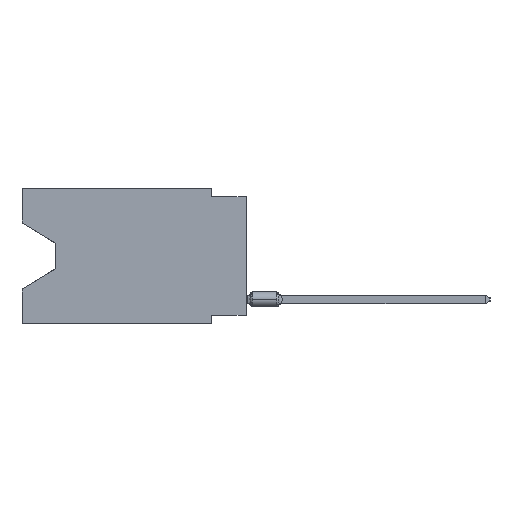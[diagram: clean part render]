
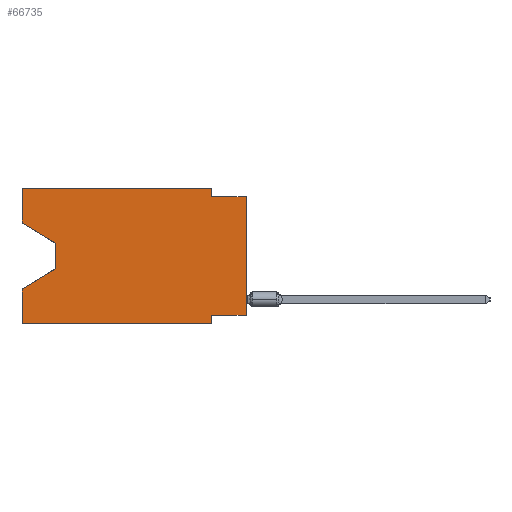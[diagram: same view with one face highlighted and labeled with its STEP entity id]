
A CAD part, left-side view. The second image highlights one B-rep face of the part: STEP entity #66735.
In plain terms, the highlighted planar face has unit normal (-1, 0, 0).
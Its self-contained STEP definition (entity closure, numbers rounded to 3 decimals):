
#975 = CARTESIAN_POINT ( 'NONE',  ( 0., 16.383, -9.906 ) ) ;
#2247 = VERTEX_POINT ( 'NONE', #31099 ) ;
#2841 = ORIENTED_EDGE ( 'NONE', *, *, #19397, .F. ) ;
#3547 = VECTOR ( 'NONE', #15946, 1000. ) ;
#5544 = VERTEX_POINT ( 'NONE', #37851 ) ;
#6447 = CARTESIAN_POINT ( 'NONE',  ( 0., 16.383, 0. ) ) ;
#9042 = LINE ( 'NONE', #21674, #3547 ) ;
#9742 = EDGE_CURVE ( 'NONE', #5544, #59320, #74086, .T. ) ;
#12204 = FACE_OUTER_BOUND ( 'NONE', #25759, .T. ) ;
#13339 = ORIENTED_EDGE ( 'NONE', *, *, #69992, .F. ) ;
#13343 = CARTESIAN_POINT ( 'NONE',  ( 0., 2.54, 0. ) ) ;
#15040 = DIRECTION ( 'NONE',  ( 0., 0., 1. ) ) ;
#15249 = CARTESIAN_POINT ( 'NONE',  ( 0., 16.383, -2.546 ) ) ;
#15946 = DIRECTION ( 'NONE',  ( 0., -1., 0. ) ) ;
#18951 = EDGE_CURVE ( 'NONE', #69883, #52022, #30192, .T. ) ;
#19292 = CARTESIAN_POINT ( 'NONE',  ( 0., 16.383, -2.546 ) ) ;
#19304 = VECTOR ( 'NONE', #20701, 1000. ) ;
#19397 = EDGE_CURVE ( 'NONE', #34182, #2247, #49482, .T. ) ;
#19448 = CARTESIAN_POINT ( 'NONE',  ( 0., 0., 0. ) ) ;
#20510 = CARTESIAN_POINT ( 'NONE',  ( 0., 16.383, 0. ) ) ;
#20682 = VECTOR ( 'NONE', #36139, 1000. ) ;
#20701 = DIRECTION ( 'NONE',  ( 0., 0.855, -0.519 ) ) ;
#21674 = CARTESIAN_POINT ( 'NONE',  ( 0., 16.383, 0. ) ) ;
#22141 = VECTOR ( 'NONE', #64685, 1000. ) ;
#22697 = ORIENTED_EDGE ( 'NONE', *, *, #55579, .F. ) ;
#23872 = VECTOR ( 'NONE', #60016, 1000. ) ;
#23886 = CARTESIAN_POINT ( 'NONE',  ( 0., 2.54, -9.906 ) ) ;
#24367 = DIRECTION ( 'NONE',  ( 0., -1., 0. ) ) ;
#25759 = EDGE_LOOP ( 'NONE', ( #30781, #75148, #58285, #2841, #42229, #50373, #13339, #27452, #71503, #27538, #65998, #22697 ) ) ;
#25778 = CARTESIAN_POINT ( 'NONE',  ( 0., 16.383, 0. ) ) ;
#26527 = DIRECTION ( 'NONE',  ( 0., 0., 1. ) ) ;
#27452 = ORIENTED_EDGE ( 'NONE', *, *, #18951, .T. ) ;
#27538 = ORIENTED_EDGE ( 'NONE', *, *, #59784, .F. ) ;
#27880 = CARTESIAN_POINT ( 'NONE',  ( 0., 0., -9.271 ) ) ;
#27900 = EDGE_CURVE ( 'NONE', #73629, #42611, #9042, .T. ) ;
#29206 = VECTOR ( 'NONE', #29652, 1000. ) ;
#29652 = DIRECTION ( 'NONE',  ( 0., -0.855, -0.519 ) ) ;
#29824 = DIRECTION ( 'NONE',  ( 1., 0., 0. ) ) ;
#29923 = CARTESIAN_POINT ( 'NONE',  ( 0., 0., -0.635 ) ) ;
#30035 = LINE ( 'NONE', #19292, #29206 ) ;
#30192 = LINE ( 'NONE', #19448, #43479 ) ;
#30781 = ORIENTED_EDGE ( 'NONE', *, *, #48621, .T. ) ;
#31099 = CARTESIAN_POINT ( 'NONE',  ( 0., 16.383, -7.36 ) ) ;
#31426 = CARTESIAN_POINT ( 'NONE',  ( 0., 13.97, -5.893 ) ) ;
#32023 = CARTESIAN_POINT ( 'NONE',  ( 0., 2.54, 0. ) ) ;
#34182 = VERTEX_POINT ( 'NONE', #67827 ) ;
#34357 = CARTESIAN_POINT ( 'NONE',  ( 0., 2.54, -9.906 ) ) ;
#35885 = DIRECTION ( 'NONE',  ( 0., 1., 0. ) ) ;
#36139 = DIRECTION ( 'NONE',  ( 0., 0., -1. ) ) ;
#37851 = CARTESIAN_POINT ( 'NONE',  ( 0., 13.97, -4.013 ) ) ;
#38012 = EDGE_CURVE ( 'NONE', #70819, #52022, #75095, .T. ) ;
#38298 = LINE ( 'NONE', #31426, #19304 ) ;
#39870 = VECTOR ( 'NONE', #15040, 1000. ) ;
#41022 = CARTESIAN_POINT ( 'NONE',  ( 0., 2.54, -9.271 ) ) ;
#41683 = DIRECTION ( 'NONE',  ( 0., 0., -1. ) ) ;
#41801 = EDGE_CURVE ( 'NONE', #34182, #57193, #59590, .T. ) ;
#42010 = CARTESIAN_POINT ( 'NONE',  ( 0., 0., -9.271 ) ) ;
#42229 = ORIENTED_EDGE ( 'NONE', *, *, #41801, .T. ) ;
#42611 = VERTEX_POINT ( 'NONE', #13343 ) ;
#43479 = VECTOR ( 'NONE', #48913, 1000. ) ;
#46321 = CARTESIAN_POINT ( 'NONE',  ( 0., 13.97, -5.893 ) ) ;
#46770 = VECTOR ( 'NONE', #24367, 1000. ) ;
#48500 = LINE ( 'NONE', #42010, #48800 ) ;
#48554 = EDGE_CURVE ( 'NONE', #68034, #57193, #65264, .T. ) ;
#48621 = EDGE_CURVE ( 'NONE', #73162, #5544, #30035, .T. ) ;
#48725 = CARTESIAN_POINT ( 'NONE',  ( 0., 16.383, 0. ) ) ;
#48800 = VECTOR ( 'NONE', #35885, 1000. ) ;
#48913 = DIRECTION ( 'NONE',  ( 0., 0., 1. ) ) ;
#49482 = LINE ( 'NONE', #48725, #39870 ) ;
#50373 = ORIENTED_EDGE ( 'NONE', *, *, #48554, .F. ) ;
#51043 = CARTESIAN_POINT ( 'NONE',  ( 0., 13.97, -4.013 ) ) ;
#52022 = VERTEX_POINT ( 'NONE', #29923 ) ;
#55008 = LINE ( 'NONE', #32023, #23872 ) ;
#55579 = EDGE_CURVE ( 'NONE', #73162, #73629, #60625, .T. ) ;
#57193 = VERTEX_POINT ( 'NONE', #34357 ) ;
#58285 = ORIENTED_EDGE ( 'NONE', *, *, #68229, .T. ) ;
#58918 = PLANE ( 'NONE',  #68091 ) ;
#59320 = VERTEX_POINT ( 'NONE', #46321 ) ;
#59590 = LINE ( 'NONE', #975, #46770 ) ;
#59784 = EDGE_CURVE ( 'NONE', #42611, #70819, #55008, .T. ) ;
#60016 = DIRECTION ( 'NONE',  ( 0., 0., -1. ) ) ;
#60625 = LINE ( 'NONE', #25778, #70172 ) ;
#63559 = CARTESIAN_POINT ( 'NONE',  ( 0., 0., -0.635 ) ) ;
#64685 = DIRECTION ( 'NONE',  ( 0., -1., 0. ) ) ;
#65194 = CARTESIAN_POINT ( 'NONE',  ( 0., 2.54, -0.635 ) ) ;
#65264 = LINE ( 'NONE', #23886, #20682 ) ;
#65998 = ORIENTED_EDGE ( 'NONE', *, *, #27900, .F. ) ;
#66735 = ADVANCED_FACE ( 'NONE', ( #12204 ), #58918, .F. ) ;
#67827 = CARTESIAN_POINT ( 'NONE',  ( 0., 16.383, -9.906 ) ) ;
#68034 = VERTEX_POINT ( 'NONE', #41022 ) ;
#68091 = AXIS2_PLACEMENT_3D ( 'NONE', #6447, #29824, #41683 ) ;
#68229 = EDGE_CURVE ( 'NONE', #59320, #2247, #38298, .T. ) ;
#68329 = VECTOR ( 'NONE', #74470, 1000. ) ;
#69883 = VERTEX_POINT ( 'NONE', #27880 ) ;
#69992 = EDGE_CURVE ( 'NONE', #69883, #68034, #48500, .T. ) ;
#70172 = VECTOR ( 'NONE', #26527, 1000. ) ;
#70819 = VERTEX_POINT ( 'NONE', #65194 ) ;
#71503 = ORIENTED_EDGE ( 'NONE', *, *, #38012, .F. ) ;
#73162 = VERTEX_POINT ( 'NONE', #15249 ) ;
#73629 = VERTEX_POINT ( 'NONE', #20510 ) ;
#74086 = LINE ( 'NONE', #51043, #68329 ) ;
#74470 = DIRECTION ( 'NONE',  ( 0., 0., -1. ) ) ;
#75095 = LINE ( 'NONE', #63559, #22141 ) ;
#75148 = ORIENTED_EDGE ( 'NONE', *, *, #9742, .T. ) ;
